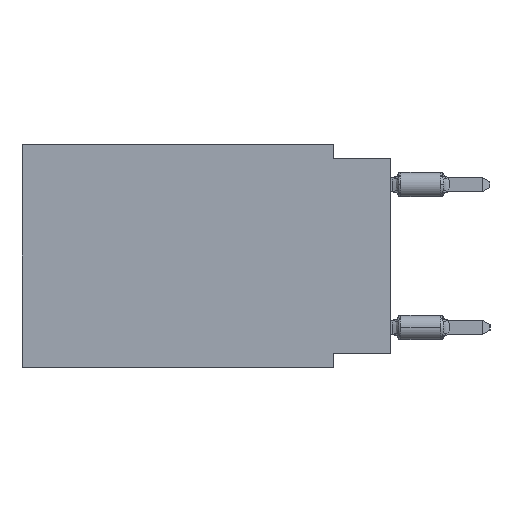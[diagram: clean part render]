
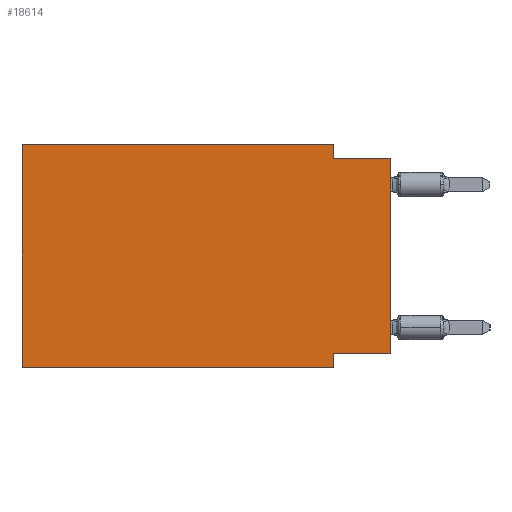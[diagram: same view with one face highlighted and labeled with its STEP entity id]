
A CAD part, left-side view. The second image highlights one B-rep face of the part: STEP entity #18614.
In plain terms, the highlighted planar face has unit normal (-1, 0, 0).
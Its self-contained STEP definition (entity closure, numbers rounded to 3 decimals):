
#365 = CARTESIAN_POINT ( 'NONE',  ( 0., 0., 0. ) ) ;
#538 = DIRECTION ( 'NONE',  ( 1., 0., 0. ) ) ;
#1245 = CARTESIAN_POINT ( 'NONE',  ( 0., 2.54, 0. ) ) ;
#1542 = LINE ( 'NONE', #4198, #7824 ) ;
#1818 = CARTESIAN_POINT ( 'NONE',  ( 0., 2.54, -9.906 ) ) ;
#2596 = CARTESIAN_POINT ( 'NONE',  ( 0., 16.383, 0. ) ) ;
#4198 = CARTESIAN_POINT ( 'NONE',  ( 0., 16.383, 0. ) ) ;
#4387 = ORIENTED_EDGE ( 'NONE', *, *, #15989, .F. ) ;
#4601 = CARTESIAN_POINT ( 'NONE',  ( 0., 16.383, -9.906 ) ) ;
#6492 = VECTOR ( 'NONE', #12735, 1000. ) ;
#7364 = CARTESIAN_POINT ( 'NONE',  ( 0., 2.54, 0. ) ) ;
#7458 = ORIENTED_EDGE ( 'NONE', *, *, #12683, .F. ) ;
#7616 = VERTEX_POINT ( 'NONE', #2596 ) ;
#7705 = ORIENTED_EDGE ( 'NONE', *, *, #20994, .F. ) ;
#7824 = VECTOR ( 'NONE', #19422, 1000. ) ;
#8415 = CARTESIAN_POINT ( 'NONE',  ( 0., 0., -0.635 ) ) ;
#8491 = PLANE ( 'NONE',  #13542 ) ;
#9282 = LINE ( 'NONE', #11942, #11057 ) ;
#10657 = LINE ( 'NONE', #365, #13573 ) ;
#10663 = DIRECTION ( 'NONE',  ( 0., 0., -1. ) ) ;
#10724 = CARTESIAN_POINT ( 'NONE',  ( 0., 16.383, 0. ) ) ;
#11057 = VECTOR ( 'NONE', #14587, 1000. ) ;
#11060 = ORIENTED_EDGE ( 'NONE', *, *, #23369, .F. ) ;
#11073 = CARTESIAN_POINT ( 'NONE',  ( 0., 16.383, -9.906 ) ) ;
#11942 = CARTESIAN_POINT ( 'NONE',  ( 0., 0., -9.271 ) ) ;
#12012 = VERTEX_POINT ( 'NONE', #28567 ) ;
#12683 = EDGE_CURVE ( 'NONE', #7616, #17285, #17863, .T. ) ;
#12735 = DIRECTION ( 'NONE',  ( 0., -1., 0. ) ) ;
#13542 = AXIS2_PLACEMENT_3D ( 'NONE', #28545, #538, #10663 ) ;
#13573 = VECTOR ( 'NONE', #28539, 1000. ) ;
#13597 = VECTOR ( 'NONE', #26614, 1000. ) ;
#13770 = VERTEX_POINT ( 'NONE', #1818 ) ;
#14587 = DIRECTION ( 'NONE',  ( 0., 1., 0. ) ) ;
#15026 = CARTESIAN_POINT ( 'NONE',  ( 0., 2.54, -9.271 ) ) ;
#15956 = VERTEX_POINT ( 'NONE', #27350 ) ;
#15989 = EDGE_CURVE ( 'NONE', #15956, #31288, #9282, .T. ) ;
#16348 = VECTOR ( 'NONE', #27989, 1000. ) ;
#17285 = VERTEX_POINT ( 'NONE', #7364 ) ;
#17361 = EDGE_CURVE ( 'NONE', #15956, #12012, #10657, .T. ) ;
#17466 = VECTOR ( 'NONE', #31414, 1000. ) ;
#17593 = EDGE_LOOP ( 'NONE', ( #25126, #31400, #11060, #7458, #7705, #31674, #32291, #4387 ) ) ;
#17863 = LINE ( 'NONE', #10724, #16348 ) ;
#18614 = ADVANCED_FACE ( 'NONE', ( #23389 ), #8491, .F. ) ;
#18785 = EDGE_CURVE ( 'NONE', #31288, #13770, #19394, .T. ) ;
#19067 = CARTESIAN_POINT ( 'NONE',  ( 0., 2.54, -9.906 ) ) ;
#19394 = LINE ( 'NONE', #19067, #27336 ) ;
#19422 = DIRECTION ( 'NONE',  ( 0., 0., 1. ) ) ;
#19490 = EDGE_CURVE ( 'NONE', #23857, #12012, #31592, .T. ) ;
#20994 = EDGE_CURVE ( 'NONE', #24518, #7616, #1542, .T. ) ;
#23369 = EDGE_CURVE ( 'NONE', #17285, #23857, #23636, .T. ) ;
#23389 = FACE_OUTER_BOUND ( 'NONE', #17593, .T. ) ;
#23636 = LINE ( 'NONE', #1245, #17466 ) ;
#23857 = VERTEX_POINT ( 'NONE', #24418 ) ;
#24418 = CARTESIAN_POINT ( 'NONE',  ( 0., 2.54, -0.635 ) ) ;
#24518 = VERTEX_POINT ( 'NONE', #11073 ) ;
#25126 = ORIENTED_EDGE ( 'NONE', *, *, #17361, .T. ) ;
#25994 = EDGE_CURVE ( 'NONE', #24518, #13770, #27297, .T. ) ;
#26614 = DIRECTION ( 'NONE',  ( 0., -1., 0. ) ) ;
#26698 = DIRECTION ( 'NONE',  ( 0., 0., -1. ) ) ;
#27297 = LINE ( 'NONE', #4601, #6492 ) ;
#27336 = VECTOR ( 'NONE', #26698, 1000. ) ;
#27350 = CARTESIAN_POINT ( 'NONE',  ( 0., 0., -9.271 ) ) ;
#27989 = DIRECTION ( 'NONE',  ( 0., -1., 0. ) ) ;
#28539 = DIRECTION ( 'NONE',  ( 0., 0., 1. ) ) ;
#28545 = CARTESIAN_POINT ( 'NONE',  ( 0., 16.383, 0. ) ) ;
#28567 = CARTESIAN_POINT ( 'NONE',  ( 0., 0., -0.635 ) ) ;
#31288 = VERTEX_POINT ( 'NONE', #15026 ) ;
#31400 = ORIENTED_EDGE ( 'NONE', *, *, #19490, .F. ) ;
#31414 = DIRECTION ( 'NONE',  ( 0., 0., -1. ) ) ;
#31592 = LINE ( 'NONE', #8415, #13597 ) ;
#31674 = ORIENTED_EDGE ( 'NONE', *, *, #25994, .T. ) ;
#32291 = ORIENTED_EDGE ( 'NONE', *, *, #18785, .F. ) ;
